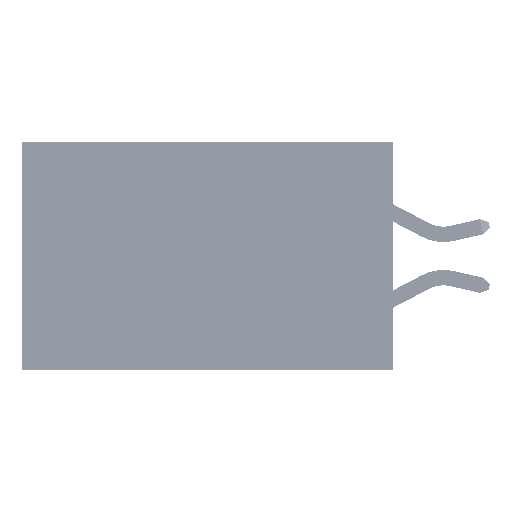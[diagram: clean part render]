
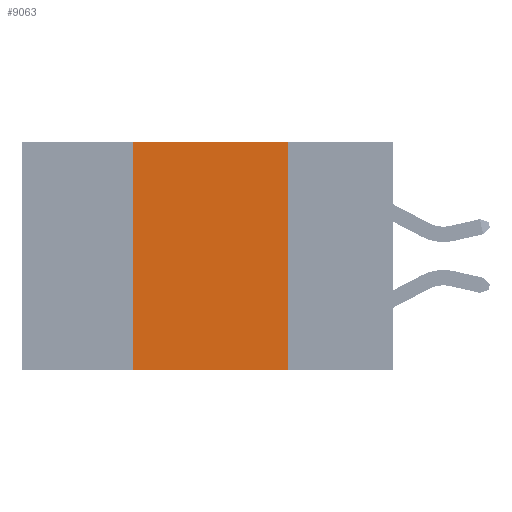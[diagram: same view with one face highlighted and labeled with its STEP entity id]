
A CAD part, left-side view. The second image highlights one B-rep face of the part: STEP entity #9063.
In plain terms, the highlighted planar face has unit normal (-1, 0, 0).
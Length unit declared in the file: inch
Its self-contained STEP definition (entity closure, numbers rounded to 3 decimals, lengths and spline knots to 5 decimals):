
#818 = EDGE_CURVE ( 'NONE', #42401, #16909, #14831, .T. ) ;
#1268 = EDGE_CURVE ( 'NONE', #30897, #23309, #15221, .T. ) ;
#3653 = DIRECTION ( 'NONE',  ( 0., 0., -1. ) ) ;
#4105 = EDGE_LOOP ( 'NONE', ( #6968, #22685, #10382, #31082 ) ) ;
#6968 = ORIENTED_EDGE ( 'NONE', *, *, #34759, .F. ) ;
#7797 = DIRECTION ( 'NONE',  ( 0., -1., 0. ) ) ;
#9063 = ADVANCED_FACE ( 'NONE', ( #28648 ), #24576, .F. ) ;
#9186 = VECTOR ( 'NONE', #13963, 39.37008 ) ;
#10382 = ORIENTED_EDGE ( 'NONE', *, *, #33821, .F. ) ;
#10744 = CARTESIAN_POINT ( 'NONE',  ( 0., 0.6, 0. ) ) ;
#10795 = CARTESIAN_POINT ( 'NONE',  ( 0., 0.42, 0. ) ) ;
#12057 = VECTOR ( 'NONE', #3653, 39.37008 ) ;
#13963 = DIRECTION ( 'NONE',  ( 0., 0., 1. ) ) ;
#14831 = LINE ( 'NONE', #35249, #15246 ) ;
#15221 = LINE ( 'NONE', #18185, #25669 ) ;
#15246 = VECTOR ( 'NONE', #7797, 39.37008 ) ;
#16909 = VERTEX_POINT ( 'NONE', #33207 ) ;
#18106 = AXIS2_PLACEMENT_3D ( 'NONE', #10744, #28211, #38648 ) ;
#18185 = CARTESIAN_POINT ( 'NONE',  ( 0., 0.6, 0. ) ) ;
#18402 = DIRECTION ( 'NONE',  ( 0., -1., 0. ) ) ;
#19901 = CARTESIAN_POINT ( 'NONE',  ( 0., 0.42, -0.37 ) ) ;
#20223 = LINE ( 'NONE', #34728, #12057 ) ;
#22685 = ORIENTED_EDGE ( 'NONE', *, *, #1268, .F. ) ;
#23309 = VERTEX_POINT ( 'NONE', #31600 ) ;
#24576 = PLANE ( 'NONE',  #18106 ) ;
#25669 = VECTOR ( 'NONE', #18402, 39.37008 ) ;
#27807 = LINE ( 'NONE', #10795, #9186 ) ;
#28211 = DIRECTION ( 'NONE',  ( 1., 0., 0. ) ) ;
#28648 = FACE_OUTER_BOUND ( 'NONE', #4105, .T. ) ;
#30897 = VERTEX_POINT ( 'NONE', #31095 ) ;
#31082 = ORIENTED_EDGE ( 'NONE', *, *, #818, .T. ) ;
#31095 = CARTESIAN_POINT ( 'NONE',  ( 0., 0.42, 0. ) ) ;
#31600 = CARTESIAN_POINT ( 'NONE',  ( 0., 0.17, 0. ) ) ;
#33207 = CARTESIAN_POINT ( 'NONE',  ( 0., 0.17, -0.37 ) ) ;
#33821 = EDGE_CURVE ( 'NONE', #42401, #30897, #27807, .T. ) ;
#34728 = CARTESIAN_POINT ( 'NONE',  ( 0., 0.17, 0. ) ) ;
#34759 = EDGE_CURVE ( 'NONE', #23309, #16909, #20223, .T. ) ;
#35249 = CARTESIAN_POINT ( 'NONE',  ( 0., 0.6, -0.37 ) ) ;
#38648 = DIRECTION ( 'NONE',  ( 0., 0., -1. ) ) ;
#42401 = VERTEX_POINT ( 'NONE', #19901 ) ;
